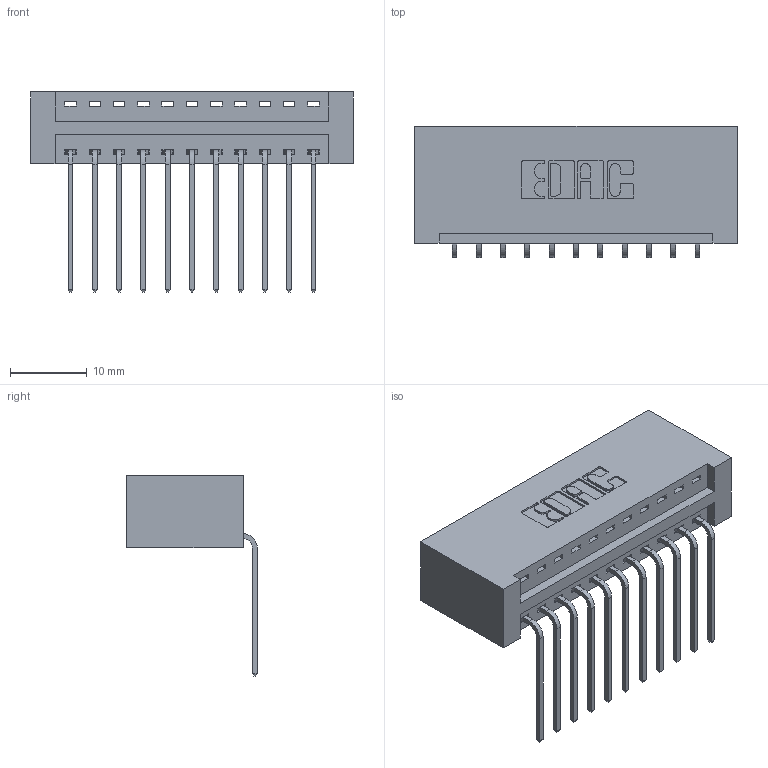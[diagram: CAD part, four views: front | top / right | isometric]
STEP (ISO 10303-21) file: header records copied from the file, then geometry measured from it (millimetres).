
FILE_DESCRIPTION (( 'STEP AP203' ), '1' );
FILE_NAME ('346-011-559-101.STEP', '2022-05-05T01:54:24', ( '' ), ( '' ), 'SwSTEP 2.0', 'SolidWorks 2020', '' );
FILE_SCHEMA (( 'CONFIG_CONTROL_DESIGN' ));
Length unit declared in the file: inch
Products named in the file (3): 346 Part_No Mounting Lugs; 345-292-001_558 559 Tail - 1; 346-011-559-101
Assembly tree (12 placements, depth 2):
  346-011-559-101
    346 Part_No Mounting Lugs
    345-292-001_558 559 Tail - 1  x11
Bounding box: 42.16 x 17.08 x 26.16 mm (x, y, z)
Volume: 4408.5 mm3; surface area: 5469.3 mm2
Topology: 12 solids, 12 shells, 774 faces, 2307 edges, 1522 vertices
Faces by surface type: plane 534, cylinder 240
Entity records: 10807 total; most frequent: CARTESIAN_POINT 1869, ORIENTED_EDGE 1814, DIRECTION 1681, EDGE_CURVE 907, VECTOR 739, LINE 739, VERTEX_POINT 602, AXIS2_PLACEMENT_3D 471
